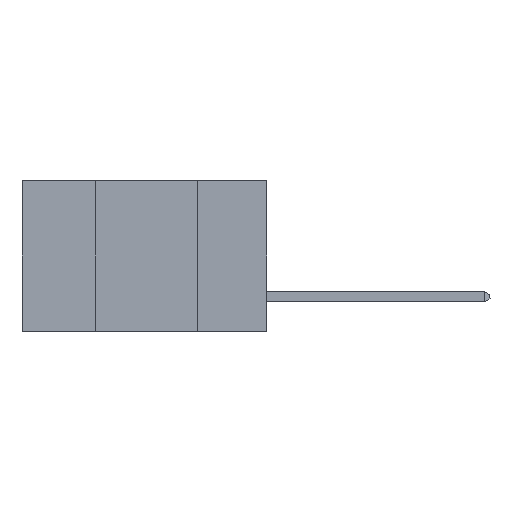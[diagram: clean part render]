
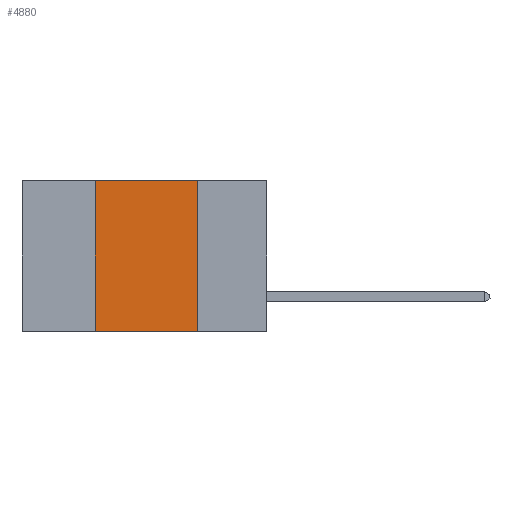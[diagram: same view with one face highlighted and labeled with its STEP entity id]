
A CAD part, left-side view. The second image highlights one B-rep face of the part: STEP entity #4880.
In plain terms, the highlighted planar face has unit normal (-1, 0, 0).
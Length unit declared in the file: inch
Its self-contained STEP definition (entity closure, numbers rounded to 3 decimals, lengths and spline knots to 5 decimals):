
#167 = CARTESIAN_POINT ( 'NONE',  ( 0., 0.42, 0. ) ) ;
#231 = ORIENTED_EDGE ( 'NONE', *, *, #3108, .F. ) ;
#353 = VECTOR ( 'NONE', #4755, 39.37008 ) ;
#587 = ORIENTED_EDGE ( 'NONE', *, *, #2812, .T. ) ;
#656 = DIRECTION ( 'NONE',  ( 0., 0., -1. ) ) ;
#1554 = CARTESIAN_POINT ( 'NONE',  ( 0., 0.6, 0. ) ) ;
#1893 = EDGE_LOOP ( 'NONE', ( #5164, #231, #8470, #587 ) ) ;
#2156 = LINE ( 'NONE', #8166, #353 ) ;
#2333 = VERTEX_POINT ( 'NONE', #3447 ) ;
#2446 = VERTEX_POINT ( 'NONE', #6414 ) ;
#2607 = DIRECTION ( 'NONE',  ( 0., -1., 0. ) ) ;
#2812 = EDGE_CURVE ( 'NONE', #6138, #2446, #5989, .T. ) ;
#2982 = CARTESIAN_POINT ( 'NONE',  ( 0., 0.42, -0.37 ) ) ;
#3040 = VERTEX_POINT ( 'NONE', #8290 ) ;
#3108 = EDGE_CURVE ( 'NONE', #3040, #2333, #4045, .T. ) ;
#3180 = VECTOR ( 'NONE', #2607, 39.37008 ) ;
#3447 = CARTESIAN_POINT ( 'NONE',  ( 0., 0.17, 0. ) ) ;
#3792 = VECTOR ( 'NONE', #7057, 39.37008 ) ;
#4045 = LINE ( 'NONE', #1554, #8901 ) ;
#4152 = DIRECTION ( 'NONE',  ( 1., 0., 0. ) ) ;
#4321 = EDGE_CURVE ( 'NONE', #6138, #3040, #8466, .T. ) ;
#4755 = DIRECTION ( 'NONE',  ( 0., 0., -1. ) ) ;
#4775 = AXIS2_PLACEMENT_3D ( 'NONE', #5317, #4152, #656 ) ;
#4880 = ADVANCED_FACE ( 'NONE', ( #4886 ), #5488, .F. ) ;
#4886 = FACE_OUTER_BOUND ( 'NONE', #1893, .T. ) ;
#5013 = DIRECTION ( 'NONE',  ( 0., -1., 0. ) ) ;
#5164 = ORIENTED_EDGE ( 'NONE', *, *, #5456, .F. ) ;
#5317 = CARTESIAN_POINT ( 'NONE',  ( 0., 0.6, 0. ) ) ;
#5456 = EDGE_CURVE ( 'NONE', #2333, #2446, #2156, .T. ) ;
#5488 = PLANE ( 'NONE',  #4775 ) ;
#5989 = LINE ( 'NONE', #6129, #3180 ) ;
#6129 = CARTESIAN_POINT ( 'NONE',  ( 0., 0.6, -0.37 ) ) ;
#6138 = VERTEX_POINT ( 'NONE', #2982 ) ;
#6414 = CARTESIAN_POINT ( 'NONE',  ( 0., 0.17, -0.37 ) ) ;
#7057 = DIRECTION ( 'NONE',  ( 0., 0., 1. ) ) ;
#8166 = CARTESIAN_POINT ( 'NONE',  ( 0., 0.17, 0. ) ) ;
#8290 = CARTESIAN_POINT ( 'NONE',  ( 0., 0.42, 0. ) ) ;
#8466 = LINE ( 'NONE', #167, #3792 ) ;
#8470 = ORIENTED_EDGE ( 'NONE', *, *, #4321, .F. ) ;
#8901 = VECTOR ( 'NONE', #5013, 39.37008 ) ;
